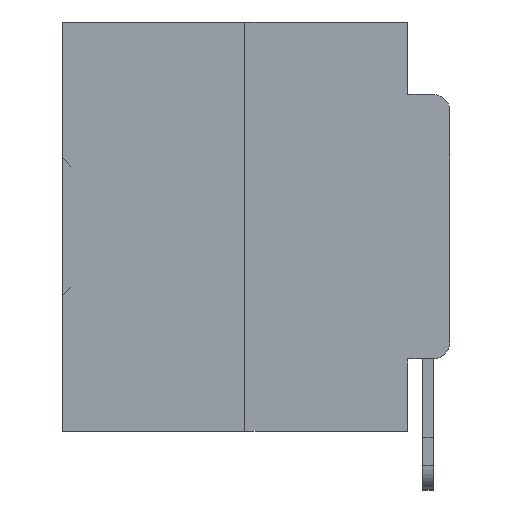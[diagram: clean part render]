
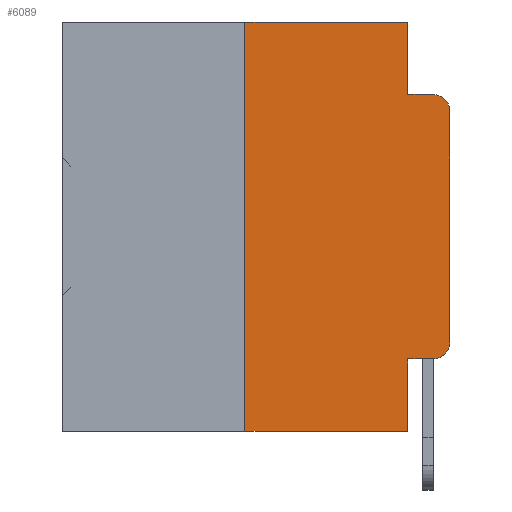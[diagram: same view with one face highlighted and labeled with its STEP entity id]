
A CAD part, left-side view. The second image highlights one B-rep face of the part: STEP entity #6089.
In plain terms, the highlighted planar face has unit normal (-1, 0, 0).
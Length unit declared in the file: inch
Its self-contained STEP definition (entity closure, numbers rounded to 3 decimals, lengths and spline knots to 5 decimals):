
#430 = CARTESIAN_POINT ( 'NONE',  ( 0., 0.051, -0.4115 ) ) ;
#627 = DIRECTION ( 'NONE',  ( 0., 0., -1. ) ) ;
#690 = VERTEX_POINT ( 'NONE', #430 ) ;
#947 = VERTEX_POINT ( 'NONE', #28896 ) ;
#1187 = LINE ( 'NONE', #18746, #8902 ) ;
#1342 = DIRECTION ( 'NONE',  ( 0., -1., 0. ) ) ;
#2218 = CARTESIAN_POINT ( 'NONE',  ( 0., 0.25, 0. ) ) ;
#3221 = VERTEX_POINT ( 'NONE', #27786 ) ;
#3785 = CARTESIAN_POINT ( 'NONE',  ( 0., 0.473, -0.5 ) ) ;
#3879 = VERTEX_POINT ( 'NONE', #25272 ) ;
#4137 = EDGE_LOOP ( 'NONE', ( #22826, #23531, #5491, #23013, #4277, #12962, #27045, #10099, #16280, #34736 ) ) ;
#4277 = ORIENTED_EDGE ( 'NONE', *, *, #31436, .F. ) ;
#4503 = PLANE ( 'NONE',  #5096 ) ;
#4967 = EDGE_CURVE ( 'NONE', #17389, #25813, #20711, .T. ) ;
#5096 = AXIS2_PLACEMENT_3D ( 'NONE', #19399, #13444, #7532 ) ;
#5203 = EDGE_CURVE ( 'NONE', #34088, #947, #33367, .T. ) ;
#5323 = CARTESIAN_POINT ( 'NONE',  ( 0., 0.051, 0. ) ) ;
#5368 = DIRECTION ( 'NONE',  ( 0., 0., 1. ) ) ;
#5491 = ORIENTED_EDGE ( 'NONE', *, *, #28440, .F. ) ;
#6089 = ADVANCED_FACE ( 'NONE', ( #19450 ), #4503, .F. ) ;
#7532 = DIRECTION ( 'NONE',  ( 0., 0., -1. ) ) ;
#8386 = CARTESIAN_POINT ( 'NONE',  ( 0., 0.25, -0.5 ) ) ;
#8434 = CARTESIAN_POINT ( 'NONE',  ( 0., 0.051, -0.0885 ) ) ;
#8902 = VECTOR ( 'NONE', #627, 39.37008 ) ;
#8970 = CIRCLE ( 'NONE', #20264, 0.02 ) ;
#9979 = DIRECTION ( 'NONE',  ( -1., 0., 0. ) ) ;
#10063 = CARTESIAN_POINT ( 'NONE',  ( 0., 0.051, -0.0885 ) ) ;
#10099 = ORIENTED_EDGE ( 'NONE', *, *, #18291, .F. ) ;
#10256 = EDGE_CURVE ( 'NONE', #34088, #11357, #13146, .T. ) ;
#10477 = VECTOR ( 'NONE', #21601, 39.37008 ) ;
#10557 = CARTESIAN_POINT ( 'NONE',  ( 0., 0.051, -0.4115 ) ) ;
#11227 = CARTESIAN_POINT ( 'NONE',  ( 0., 0.02, -0.4115 ) ) ;
#11309 = DIRECTION ( 'NONE',  ( 0., 0., 1. ) ) ;
#11317 = CARTESIAN_POINT ( 'NONE',  ( 0., 0.02, -0.1085 ) ) ;
#11357 = VERTEX_POINT ( 'NONE', #22539 ) ;
#12857 = VECTOR ( 'NONE', #11309, 39.37008 ) ;
#12958 = AXIS2_PLACEMENT_3D ( 'NONE', #11317, #31416, #14367 ) ;
#12962 = ORIENTED_EDGE ( 'NONE', *, *, #10256, .F. ) ;
#13079 = DIRECTION ( 'NONE',  ( 0., -1., 0. ) ) ;
#13146 = LINE ( 'NONE', #2218, #26704 ) ;
#13444 = DIRECTION ( 'NONE',  ( 1., 0., 0. ) ) ;
#13877 = LINE ( 'NONE', #10557, #35559 ) ;
#14367 = DIRECTION ( 'NONE',  ( 0., 0., -1. ) ) ;
#15530 = VECTOR ( 'NONE', #13079, 39.37008 ) ;
#15794 = CARTESIAN_POINT ( 'NONE',  ( 0., 0., -0.3915 ) ) ;
#16280 = ORIENTED_EDGE ( 'NONE', *, *, #25915, .T. ) ;
#17389 = VERTEX_POINT ( 'NONE', #15794 ) ;
#18291 = EDGE_CURVE ( 'NONE', #690, #947, #28933, .T. ) ;
#18321 = VERTEX_POINT ( 'NONE', #8434 ) ;
#18746 = CARTESIAN_POINT ( 'NONE',  ( 0., 0.051, 0. ) ) ;
#18993 = EDGE_CURVE ( 'NONE', #25813, #3879, #25855, .T. ) ;
#19136 = CARTESIAN_POINT ( 'NONE',  ( 0., 0., -0.1085 ) ) ;
#19399 = CARTESIAN_POINT ( 'NONE',  ( 0., 0.473, 0. ) ) ;
#19450 = FACE_OUTER_BOUND ( 'NONE', #4137, .T. ) ;
#20264 = AXIS2_PLACEMENT_3D ( 'NONE', #27389, #9979, #30155 ) ;
#20652 = CARTESIAN_POINT ( 'NONE',  ( 0., 0.473, 0. ) ) ;
#20711 = LINE ( 'NONE', #23000, #12857 ) ;
#21601 = DIRECTION ( 'NONE',  ( 0., -1., 0. ) ) ;
#22322 = LINE ( 'NONE', #10063, #15530 ) ;
#22539 = CARTESIAN_POINT ( 'NONE',  ( 0., 0.25, 0. ) ) ;
#22826 = ORIENTED_EDGE ( 'NONE', *, *, #4967, .T. ) ;
#23000 = CARTESIAN_POINT ( 'NONE',  ( 0., 0., 0. ) ) ;
#23013 = ORIENTED_EDGE ( 'NONE', *, *, #35812, .F. ) ;
#23531 = ORIENTED_EDGE ( 'NONE', *, *, #18993, .T. ) ;
#24814 = VERTEX_POINT ( 'NONE', #11227 ) ;
#25272 = CARTESIAN_POINT ( 'NONE',  ( 0., 0.02, -0.0885 ) ) ;
#25378 = LINE ( 'NONE', #20652, #31910 ) ;
#25813 = VERTEX_POINT ( 'NONE', #19136 ) ;
#25855 = CIRCLE ( 'NONE', #12958, 0.02 ) ;
#25915 = EDGE_CURVE ( 'NONE', #690, #24814, #13877, .T. ) ;
#26704 = VECTOR ( 'NONE', #5368, 39.37008 ) ;
#27045 = ORIENTED_EDGE ( 'NONE', *, *, #5203, .T. ) ;
#27389 = CARTESIAN_POINT ( 'NONE',  ( 0., 0.02, -0.3915 ) ) ;
#27750 = EDGE_CURVE ( 'NONE', #24814, #17389, #8970, .T. ) ;
#27786 = CARTESIAN_POINT ( 'NONE',  ( 0., 0.051, 0. ) ) ;
#28440 = EDGE_CURVE ( 'NONE', #18321, #3879, #22322, .T. ) ;
#28635 = DIRECTION ( 'NONE',  ( 0., 0., -1. ) ) ;
#28896 = CARTESIAN_POINT ( 'NONE',  ( 0., 0.051, -0.5 ) ) ;
#28933 = LINE ( 'NONE', #5323, #34556 ) ;
#30155 = DIRECTION ( 'NONE',  ( 0., 0., -1. ) ) ;
#31416 = DIRECTION ( 'NONE',  ( -1., 0., 0. ) ) ;
#31436 = EDGE_CURVE ( 'NONE', #11357, #3221, #25378, .T. ) ;
#31910 = VECTOR ( 'NONE', #34547, 39.37008 ) ;
#33367 = LINE ( 'NONE', #3785, #10477 ) ;
#34088 = VERTEX_POINT ( 'NONE', #8386 ) ;
#34547 = DIRECTION ( 'NONE',  ( 0., -1., 0. ) ) ;
#34556 = VECTOR ( 'NONE', #28635, 39.37008 ) ;
#34736 = ORIENTED_EDGE ( 'NONE', *, *, #27750, .T. ) ;
#35559 = VECTOR ( 'NONE', #1342, 39.37008 ) ;
#35812 = EDGE_CURVE ( 'NONE', #3221, #18321, #1187, .T. ) ;
